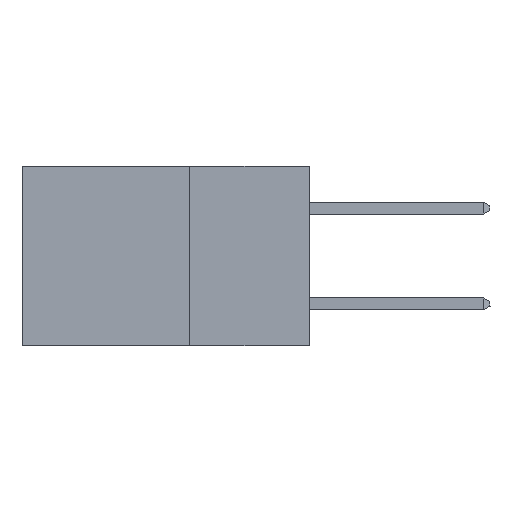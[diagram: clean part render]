
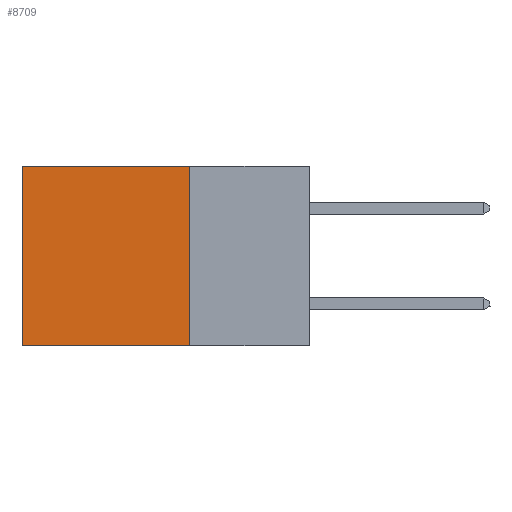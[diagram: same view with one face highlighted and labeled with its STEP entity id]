
A CAD part, left-side view. The second image highlights one B-rep face of the part: STEP entity #8709.
In plain terms, the highlighted planar face has unit normal (-1, 0, 0).
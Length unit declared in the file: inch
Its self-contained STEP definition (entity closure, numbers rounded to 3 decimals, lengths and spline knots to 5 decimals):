
#222 = DIRECTION ( 'NONE',  ( 0., 0., -1. ) ) ;
#253 = CARTESIAN_POINT ( 'NONE',  ( 0.2875, 0.25, -0.375 ) ) ;
#2845 = CARTESIAN_POINT ( 'NONE',  ( 0.2875, 0.6, -0.375 ) ) ;
#3038 = EDGE_CURVE ( 'NONE', #8766, #7005, #14805, .T. ) ;
#3762 = VECTOR ( 'NONE', #6104, 39.37008 ) ;
#5579 = VERTEX_POINT ( 'NONE', #13039 ) ;
#5619 = ORIENTED_EDGE ( 'NONE', *, *, #15565, .T. ) ;
#6104 = DIRECTION ( 'NONE',  ( 0., 0., -1. ) ) ;
#6304 = CARTESIAN_POINT ( 'NONE',  ( 0.2875, 0.25, 0. ) ) ;
#7005 = VERTEX_POINT ( 'NONE', #10172 ) ;
#7443 = CARTESIAN_POINT ( 'NONE',  ( 0.2875, 0.25, 0. ) ) ;
#8263 = CARTESIAN_POINT ( 'NONE',  ( 0.2875, 0.25, -0.375 ) ) ;
#8709 = ADVANCED_FACE ( 'NONE', ( #14453 ), #15704, .F. ) ;
#8766 = VERTEX_POINT ( 'NONE', #6304 ) ;
#8881 = LINE ( 'NONE', #9960, #13411 ) ;
#9680 = EDGE_CURVE ( 'NONE', #8766, #11190, #17552, .T. ) ;
#9779 = VECTOR ( 'NONE', #18413, 39.37008 ) ;
#9847 = EDGE_CURVE ( 'NONE', #11190, #5579, #8881, .T. ) ;
#9861 = VECTOR ( 'NONE', #222, 39.37008 ) ;
#9960 = CARTESIAN_POINT ( 'NONE',  ( 0.2875, 0.25, -0.375 ) ) ;
#10172 = CARTESIAN_POINT ( 'NONE',  ( 0.2875, 0.6, 0. ) ) ;
#11190 = VERTEX_POINT ( 'NONE', #8263 ) ;
#11266 = ORIENTED_EDGE ( 'NONE', *, *, #9680, .F. ) ;
#11454 = EDGE_LOOP ( 'NONE', ( #5619, #19647, #11266, #14687 ) ) ;
#13039 = CARTESIAN_POINT ( 'NONE',  ( 0.2875, 0.6, -0.375 ) ) ;
#13411 = VECTOR ( 'NONE', #16148, 39.37008 ) ;
#13920 = CARTESIAN_POINT ( 'NONE',  ( 0.2875, 0.25, -0.375 ) ) ;
#14137 = DIRECTION ( 'NONE',  ( 1., 0., 0. ) ) ;
#14273 = DIRECTION ( 'NONE',  ( 0., 0., -1. ) ) ;
#14453 = FACE_OUTER_BOUND ( 'NONE', #11454, .T. ) ;
#14687 = ORIENTED_EDGE ( 'NONE', *, *, #3038, .T. ) ;
#14805 = LINE ( 'NONE', #7443, #9779 ) ;
#15565 = EDGE_CURVE ( 'NONE', #7005, #5579, #19708, .T. ) ;
#15704 = PLANE ( 'NONE',  #16254 ) ;
#16148 = DIRECTION ( 'NONE',  ( 0., 1., 0. ) ) ;
#16254 = AXIS2_PLACEMENT_3D ( 'NONE', #253, #14137, #14273 ) ;
#17552 = LINE ( 'NONE', #13920, #9861 ) ;
#18413 = DIRECTION ( 'NONE',  ( 0., 1., 0. ) ) ;
#19647 = ORIENTED_EDGE ( 'NONE', *, *, #9847, .F. ) ;
#19708 = LINE ( 'NONE', #2845, #3762 ) ;
